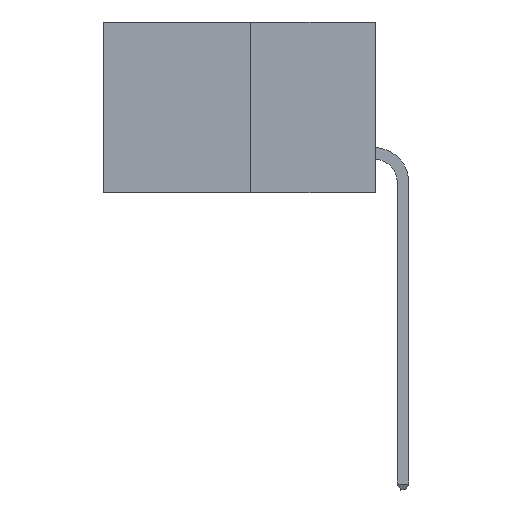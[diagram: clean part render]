
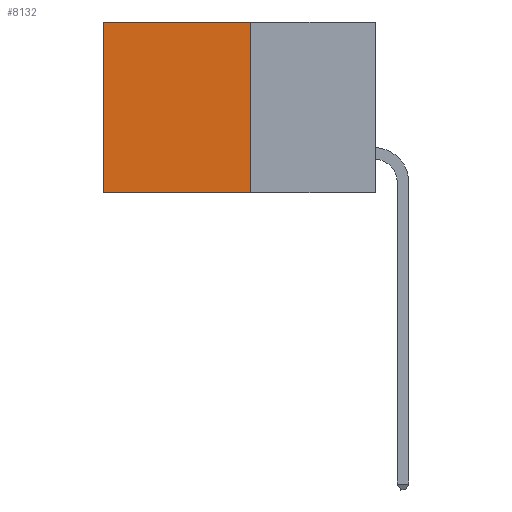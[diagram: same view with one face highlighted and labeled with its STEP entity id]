
A CAD part, left-side view. The second image highlights one B-rep face of the part: STEP entity #8132.
In plain terms, the highlighted planar face has unit normal (-1, 0, 0).
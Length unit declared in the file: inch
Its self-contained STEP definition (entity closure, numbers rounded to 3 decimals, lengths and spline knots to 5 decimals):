
#153 = LINE ( 'NONE', #9273, #9078 ) ;
#620 = ORIENTED_EDGE ( 'NONE', *, *, #2533, .F. ) ;
#681 = ORIENTED_EDGE ( 'NONE', *, *, #3729, .F. ) ;
#1063 = CARTESIAN_POINT ( 'NONE',  ( 0.277, 0.27, 0. ) ) ;
#1346 = ORIENTED_EDGE ( 'NONE', *, *, #5182, .T. ) ;
#1956 = CARTESIAN_POINT ( 'NONE',  ( 0.277, 0.59, 0. ) ) ;
#2095 = ORIENTED_EDGE ( 'NONE', *, *, #11058, .T. ) ;
#2533 = EDGE_CURVE ( 'NONE', #5285, #9861, #10038, .T. ) ;
#3475 = FACE_OUTER_BOUND ( 'NONE', #8776, .T. ) ;
#3729 = EDGE_CURVE ( 'NONE', #10784, #5285, #10885, .T. ) ;
#5182 = EDGE_CURVE ( 'NONE', #10784, #5613, #153, .T. ) ;
#5285 = VERTEX_POINT ( 'NONE', #6478 ) ;
#5613 = VERTEX_POINT ( 'NONE', #1956 ) ;
#5781 = CARTESIAN_POINT ( 'NONE',  ( 0.277, 0.27, -0.37 ) ) ;
#6403 = CARTESIAN_POINT ( 'NONE',  ( 0.277, 0.59, -0.37 ) ) ;
#6475 = LINE ( 'NONE', #9141, #10720 ) ;
#6478 = CARTESIAN_POINT ( 'NONE',  ( 0.277, 0.27, -0.37 ) ) ;
#6574 = AXIS2_PLACEMENT_3D ( 'NONE', #8786, #8287, #8036 ) ;
#6978 = DIRECTION ( 'NONE',  ( 0., 0., -1. ) ) ;
#7814 = VECTOR ( 'NONE', #9891, 39.37008 ) ;
#8036 = DIRECTION ( 'NONE',  ( 0., 0., -1. ) ) ;
#8132 = ADVANCED_FACE ( 'NONE', ( #3475 ), #8478, .F. ) ;
#8287 = DIRECTION ( 'NONE',  ( 1., 0., 0. ) ) ;
#8478 = PLANE ( 'NONE',  #6574 ) ;
#8776 = EDGE_LOOP ( 'NONE', ( #2095, #620, #681, #1346 ) ) ;
#8786 = CARTESIAN_POINT ( 'NONE',  ( 0.277, 0.27, -0.37 ) ) ;
#8838 = DIRECTION ( 'NONE',  ( 0., 1., 0. ) ) ;
#9004 = VECTOR ( 'NONE', #6978, 39.37008 ) ;
#9078 = VECTOR ( 'NONE', #8838, 39.37008 ) ;
#9141 = CARTESIAN_POINT ( 'NONE',  ( 0.277, 0.59, -0.37 ) ) ;
#9273 = CARTESIAN_POINT ( 'NONE',  ( 0.277, 0.27, 0. ) ) ;
#9861 = VERTEX_POINT ( 'NONE', #6403 ) ;
#9891 = DIRECTION ( 'NONE',  ( 0., 1., 0. ) ) ;
#9943 = DIRECTION ( 'NONE',  ( 0., 0., -1. ) ) ;
#10038 = LINE ( 'NONE', #10127, #7814 ) ;
#10127 = CARTESIAN_POINT ( 'NONE',  ( 0.277, 0.27, -0.37 ) ) ;
#10720 = VECTOR ( 'NONE', #9943, 39.37008 ) ;
#10784 = VERTEX_POINT ( 'NONE', #1063 ) ;
#10885 = LINE ( 'NONE', #5781, #9004 ) ;
#11058 = EDGE_CURVE ( 'NONE', #5613, #9861, #6475, .T. ) ;
